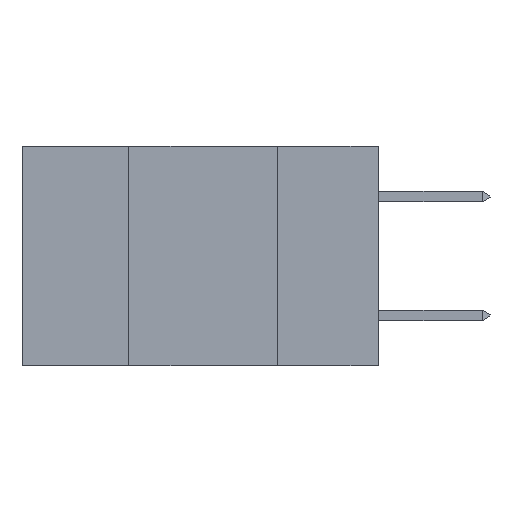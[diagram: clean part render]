
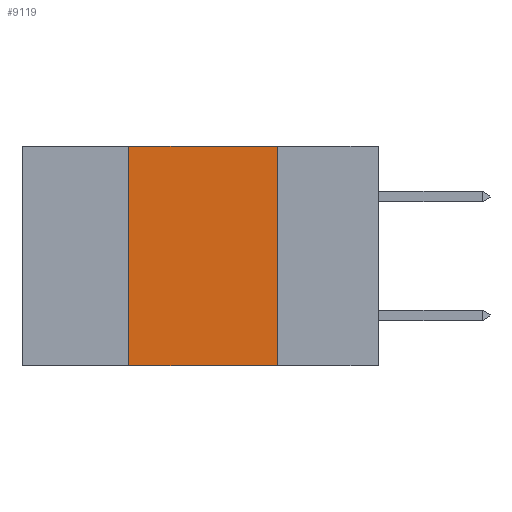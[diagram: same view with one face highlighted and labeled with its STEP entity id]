
A CAD part, left-side view. The second image highlights one B-rep face of the part: STEP entity #9119.
In plain terms, the highlighted planar face has unit normal (-1, 0, 0).
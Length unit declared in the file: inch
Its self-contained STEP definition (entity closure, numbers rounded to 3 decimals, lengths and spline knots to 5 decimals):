
#1360 = DIRECTION ( 'NONE',  ( 0., 0., -1. ) ) ;
#1721 = VERTEX_POINT ( 'NONE', #12671 ) ;
#1766 = EDGE_CURVE ( 'NONE', #10527, #1721, #14681, .T. ) ;
#2564 = CARTESIAN_POINT ( 'NONE',  ( 0., 0.17, 0. ) ) ;
#2639 = DIRECTION ( 'NONE',  ( 1., 0., 0. ) ) ;
#2698 = VECTOR ( 'NONE', #14508, 39.37008 ) ;
#3180 = FACE_OUTER_BOUND ( 'NONE', #3666, .T. ) ;
#3666 = EDGE_LOOP ( 'NONE', ( #4517, #12092, #3892, #14170 ) ) ;
#3868 = VERTEX_POINT ( 'NONE', #4613 ) ;
#3892 = ORIENTED_EDGE ( 'NONE', *, *, #12770, .F. ) ;
#4517 = ORIENTED_EDGE ( 'NONE', *, *, #1766, .F. ) ;
#4613 = CARTESIAN_POINT ( 'NONE',  ( 0., 0.42, -0.37 ) ) ;
#4980 = VECTOR ( 'NONE', #12452, 39.37008 ) ;
#5487 = VECTOR ( 'NONE', #10738, 39.37008 ) ;
#5510 = AXIS2_PLACEMENT_3D ( 'NONE', #6180, #2639, #1360 ) ;
#5744 = CARTESIAN_POINT ( 'NONE',  ( 0., 0.42, 0. ) ) ;
#5923 = VECTOR ( 'NONE', #7840, 39.37008 ) ;
#6180 = CARTESIAN_POINT ( 'NONE',  ( 0., 0.6, 0. ) ) ;
#6827 = CARTESIAN_POINT ( 'NONE',  ( 0., 0.6, 0. ) ) ;
#7840 = DIRECTION ( 'NONE',  ( 0., 0., 1. ) ) ;
#7930 = EDGE_CURVE ( 'NONE', #3868, #1721, #9971, .T. ) ;
#8242 = PLANE ( 'NONE',  #5510 ) ;
#8712 = LINE ( 'NONE', #6827, #4980 ) ;
#8911 = LINE ( 'NONE', #13466, #5923 ) ;
#9119 = ADVANCED_FACE ( 'NONE', ( #3180 ), #8242, .F. ) ;
#9971 = LINE ( 'NONE', #10122, #2698 ) ;
#10122 = CARTESIAN_POINT ( 'NONE',  ( 0., 0.6, -0.37 ) ) ;
#10527 = VERTEX_POINT ( 'NONE', #13426 ) ;
#10738 = DIRECTION ( 'NONE',  ( 0., 0., -1. ) ) ;
#12092 = ORIENTED_EDGE ( 'NONE', *, *, #14479, .F. ) ;
#12452 = DIRECTION ( 'NONE',  ( 0., -1., 0. ) ) ;
#12671 = CARTESIAN_POINT ( 'NONE',  ( 0., 0.17, -0.37 ) ) ;
#12770 = EDGE_CURVE ( 'NONE', #3868, #12917, #8911, .T. ) ;
#12917 = VERTEX_POINT ( 'NONE', #5744 ) ;
#13426 = CARTESIAN_POINT ( 'NONE',  ( 0., 0.17, 0. ) ) ;
#13466 = CARTESIAN_POINT ( 'NONE',  ( 0., 0.42, 0. ) ) ;
#14170 = ORIENTED_EDGE ( 'NONE', *, *, #7930, .T. ) ;
#14479 = EDGE_CURVE ( 'NONE', #12917, #10527, #8712, .T. ) ;
#14508 = DIRECTION ( 'NONE',  ( 0., -1., 0. ) ) ;
#14681 = LINE ( 'NONE', #2564, #5487 ) ;
